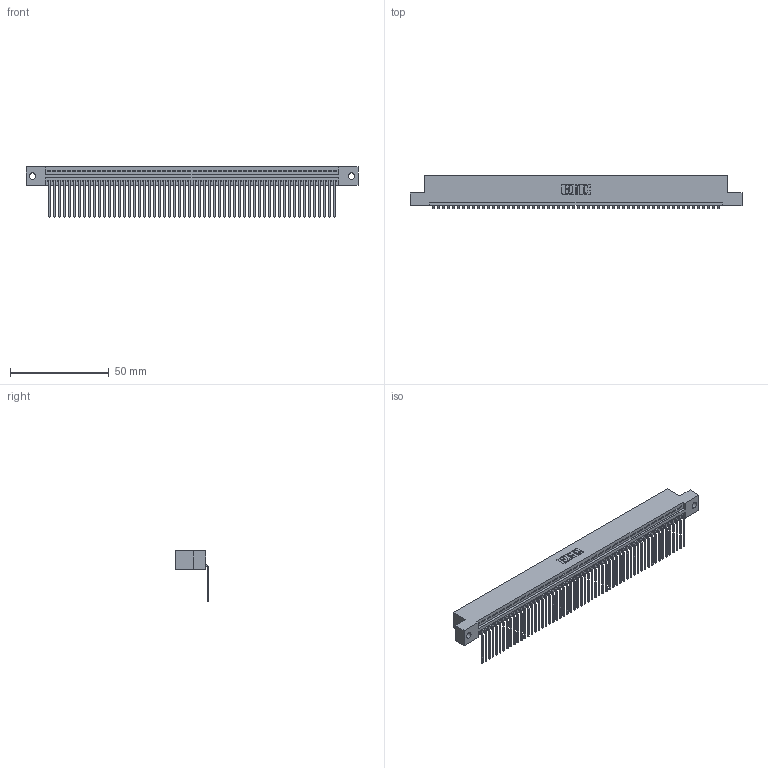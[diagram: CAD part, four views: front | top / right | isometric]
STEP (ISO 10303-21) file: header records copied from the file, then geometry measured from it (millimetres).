
FILE_DESCRIPTION (( 'STEP AP203' ), '1' );
FILE_NAME ('345-058-559-102.STEP', '2019-10-10T18:10:24', ( '' ), ( '' ), 'SwSTEP 2.0', 'SolidWorks 2016', '' );
FILE_SCHEMA (( 'CONFIG_CONTROL_DESIGN' ));
Length unit declared in the file: inch
Products named in the file (3): 345 Part_Flush Mounting Lugs - 0.128 Dia; 345-292-001_558 559 Tail - 1; 345-058-559-102
Assembly tree (59 placements, depth 2):
  345-058-559-102
    345 Part_Flush Mounting Lugs - 0.128 Dia
    345-292-001_558 559 Tail - 1  x58
Bounding box: 168.53 x 16.75 x 25.53 mm (x, y, z)
Volume: 16294.7 mm3; surface area: 22735.6 mm2
Topology: 59 solids, 59 shells, 3606 faces, 10897 edges, 7186 vertices
Faces by surface type: plane 2516, cylinder 1090
Entity records: 41585 total; most frequent: CARTESIAN_POINT 7210, ORIENTED_EDGE 7202, DIRECTION 6273, EDGE_CURVE 3601, VECTOR 3237, LINE 3237, VERTEX_POINT 2398, AXIS2_PLACEMENT_3D 1518
